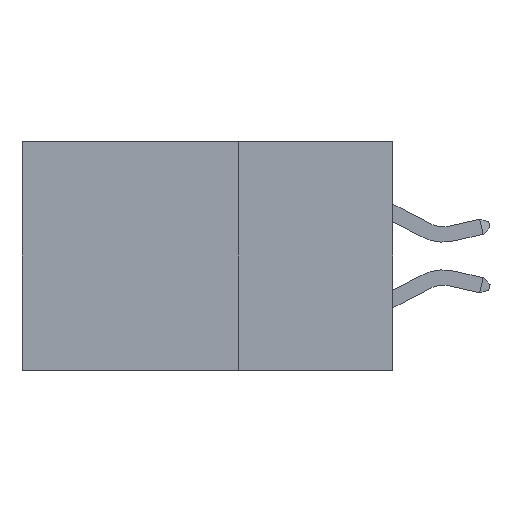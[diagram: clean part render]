
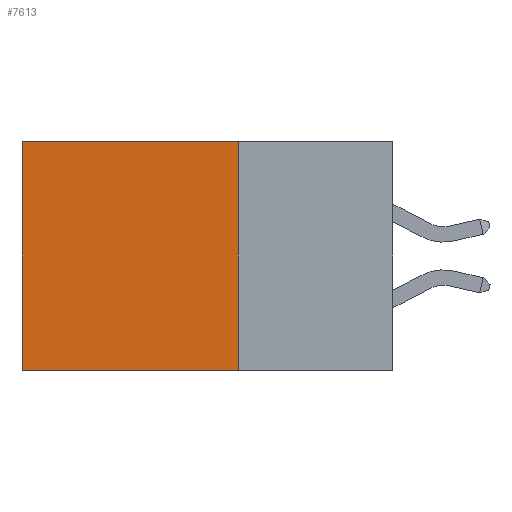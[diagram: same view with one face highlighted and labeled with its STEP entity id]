
A CAD part, left-side view. The second image highlights one B-rep face of the part: STEP entity #7613.
In plain terms, the highlighted planar face has unit normal (-1, 0, 0).
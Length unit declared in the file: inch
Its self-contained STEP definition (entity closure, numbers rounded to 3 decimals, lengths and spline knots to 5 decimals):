
#247 = DIRECTION ( 'NONE',  ( 0., 1., 0. ) ) ;
#1636 = CARTESIAN_POINT ( 'NONE',  ( 0.2875, 0.25, 0. ) ) ;
#1740 = VECTOR ( 'NONE', #10869, 39.37008 ) ;
#1743 = CARTESIAN_POINT ( 'NONE',  ( 0.2875, 0.25, 0. ) ) ;
#2166 = VECTOR ( 'NONE', #247, 39.37008 ) ;
#2493 = LINE ( 'NONE', #4081, #1740 ) ;
#2698 = EDGE_CURVE ( 'NONE', #11015, #26742, #17597, .T. ) ;
#4081 = CARTESIAN_POINT ( 'NONE',  ( 0.2875, 0.25, -0.37 ) ) ;
#4292 = VERTEX_POINT ( 'NONE', #31602 ) ;
#4301 = PLANE ( 'NONE',  #18297 ) ;
#6412 = ORIENTED_EDGE ( 'NONE', *, *, #12191, .T. ) ;
#7048 = EDGE_LOOP ( 'NONE', ( #31578, #27892, #21915, #6412 ) ) ;
#7613 = ADVANCED_FACE ( 'NONE', ( #18970 ), #4301, .F. ) ;
#10869 = DIRECTION ( 'NONE',  ( 0., 1., 0. ) ) ;
#11015 = VERTEX_POINT ( 'NONE', #21799 ) ;
#11435 = CARTESIAN_POINT ( 'NONE',  ( 0.2875, 0.6, -0.37 ) ) ;
#11544 = DIRECTION ( 'NONE',  ( 0., 0., -1. ) ) ;
#12191 = EDGE_CURVE ( 'NONE', #18576, #11015, #18237, .T. ) ;
#12813 = EDGE_CURVE ( 'NONE', #18576, #4292, #16301, .T. ) ;
#13265 = CARTESIAN_POINT ( 'NONE',  ( 0.2875, 0.6, 0. ) ) ;
#16301 = LINE ( 'NONE', #1636, #19023 ) ;
#17597 = LINE ( 'NONE', #13265, #27222 ) ;
#18237 = LINE ( 'NONE', #29591, #2166 ) ;
#18297 = AXIS2_PLACEMENT_3D ( 'NONE', #1743, #23772, #11544 ) ;
#18576 = VERTEX_POINT ( 'NONE', #27688 ) ;
#18970 = FACE_OUTER_BOUND ( 'NONE', #7048, .T. ) ;
#19023 = VECTOR ( 'NONE', #20895, 39.37008 ) ;
#20895 = DIRECTION ( 'NONE',  ( 0., 0., -1. ) ) ;
#21799 = CARTESIAN_POINT ( 'NONE',  ( 0.2875, 0.6, 0. ) ) ;
#21915 = ORIENTED_EDGE ( 'NONE', *, *, #12813, .F. ) ;
#23015 = DIRECTION ( 'NONE',  ( 0., 0., -1. ) ) ;
#23367 = EDGE_CURVE ( 'NONE', #4292, #26742, #2493, .T. ) ;
#23772 = DIRECTION ( 'NONE',  ( 1., 0., 0. ) ) ;
#26742 = VERTEX_POINT ( 'NONE', #11435 ) ;
#27222 = VECTOR ( 'NONE', #23015, 39.37008 ) ;
#27688 = CARTESIAN_POINT ( 'NONE',  ( 0.2875, 0.25, 0. ) ) ;
#27892 = ORIENTED_EDGE ( 'NONE', *, *, #23367, .F. ) ;
#29591 = CARTESIAN_POINT ( 'NONE',  ( 0.2875, 0.25, 0. ) ) ;
#31578 = ORIENTED_EDGE ( 'NONE', *, *, #2698, .T. ) ;
#31602 = CARTESIAN_POINT ( 'NONE',  ( 0.2875, 0.25, -0.37 ) ) ;
